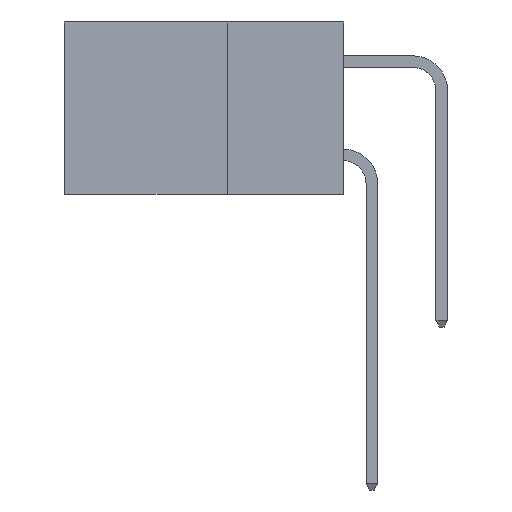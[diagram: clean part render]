
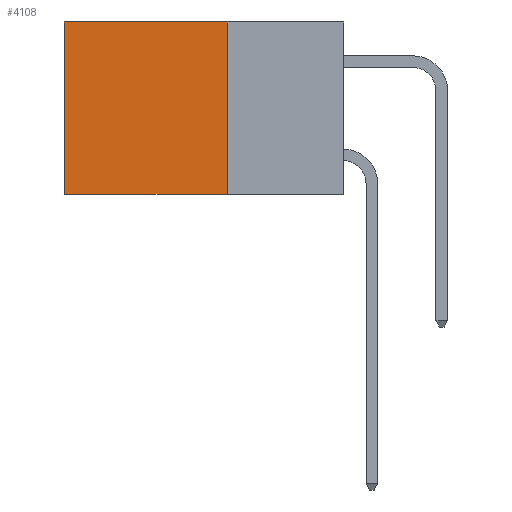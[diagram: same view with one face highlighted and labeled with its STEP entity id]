
A CAD part, left-side view. The second image highlights one B-rep face of the part: STEP entity #4108.
In plain terms, the highlighted planar face has unit normal (-1, 0, 0).
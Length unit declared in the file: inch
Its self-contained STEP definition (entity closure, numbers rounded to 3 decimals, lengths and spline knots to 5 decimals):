
#99 = EDGE_CURVE ( 'NONE', #8653, #5108, #310, .T. ) ;
#169 = VECTOR ( 'NONE', #4252, 39.37008 ) ;
#310 = LINE ( 'NONE', #10304, #169 ) ;
#511 = ORIENTED_EDGE ( 'NONE', *, *, #99, .T. ) ;
#1764 = CARTESIAN_POINT ( 'NONE',  ( 0.2615, 0.6, 0. ) ) ;
#2421 = CARTESIAN_POINT ( 'NONE',  ( 0.2615, 0.6, -0.37 ) ) ;
#2779 = LINE ( 'NONE', #5306, #8296 ) ;
#3067 = DIRECTION ( 'NONE',  ( 0., 1., 0. ) ) ;
#3079 = ORIENTED_EDGE ( 'NONE', *, *, #11463, .F. ) ;
#3164 = CARTESIAN_POINT ( 'NONE',  ( 0.2615, 0.25, -0.37 ) ) ;
#4108 = ADVANCED_FACE ( 'NONE', ( #13401 ), #6282, .F. ) ;
#4242 = VERTEX_POINT ( 'NONE', #2421 ) ;
#4252 = DIRECTION ( 'NONE',  ( 0., 1., 0. ) ) ;
#5053 = DIRECTION ( 'NONE',  ( 0., 0., -1. ) ) ;
#5108 = VERTEX_POINT ( 'NONE', #1764 ) ;
#5113 = CARTESIAN_POINT ( 'NONE',  ( 0.2615, 0.25, 0. ) ) ;
#5277 = ORIENTED_EDGE ( 'NONE', *, *, #13069, .F. ) ;
#5306 = CARTESIAN_POINT ( 'NONE',  ( 0.2615, 0.6, -0.37 ) ) ;
#5504 = LINE ( 'NONE', #3164, #11039 ) ;
#5626 = DIRECTION ( 'NONE',  ( 0., 0., -1. ) ) ;
#5642 = DIRECTION ( 'NONE',  ( 1., 0., 0. ) ) ;
#5689 = CARTESIAN_POINT ( 'NONE',  ( 0.2615, 0.25, -0.37 ) ) ;
#5860 = CARTESIAN_POINT ( 'NONE',  ( 0.2615, 0.25, -0.37 ) ) ;
#5895 = LINE ( 'NONE', #9990, #8896 ) ;
#6282 = PLANE ( 'NONE',  #8259 ) ;
#8259 = AXIS2_PLACEMENT_3D ( 'NONE', #5689, #5642, #5626 ) ;
#8296 = VECTOR ( 'NONE', #5053, 39.37008 ) ;
#8653 = VERTEX_POINT ( 'NONE', #5113 ) ;
#8896 = VECTOR ( 'NONE', #11782, 39.37008 ) ;
#9247 = ORIENTED_EDGE ( 'NONE', *, *, #13284, .T. ) ;
#9990 = CARTESIAN_POINT ( 'NONE',  ( 0.2615, 0.25, -0.37 ) ) ;
#10125 = EDGE_LOOP ( 'NONE', ( #9247, #5277, #3079, #511 ) ) ;
#10304 = CARTESIAN_POINT ( 'NONE',  ( 0.2615, 0.25, 0. ) ) ;
#11039 = VECTOR ( 'NONE', #3067, 39.37008 ) ;
#11463 = EDGE_CURVE ( 'NONE', #8653, #12133, #5895, .T. ) ;
#11782 = DIRECTION ( 'NONE',  ( 0., 0., -1. ) ) ;
#12133 = VERTEX_POINT ( 'NONE', #5860 ) ;
#13069 = EDGE_CURVE ( 'NONE', #12133, #4242, #5504, .T. ) ;
#13284 = EDGE_CURVE ( 'NONE', #5108, #4242, #2779, .T. ) ;
#13401 = FACE_OUTER_BOUND ( 'NONE', #10125, .T. ) ;
